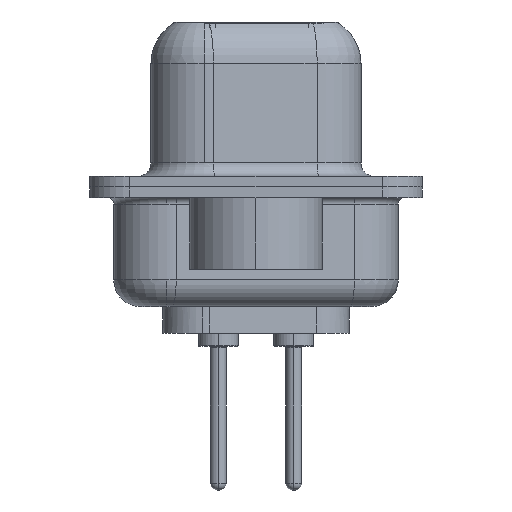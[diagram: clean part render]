
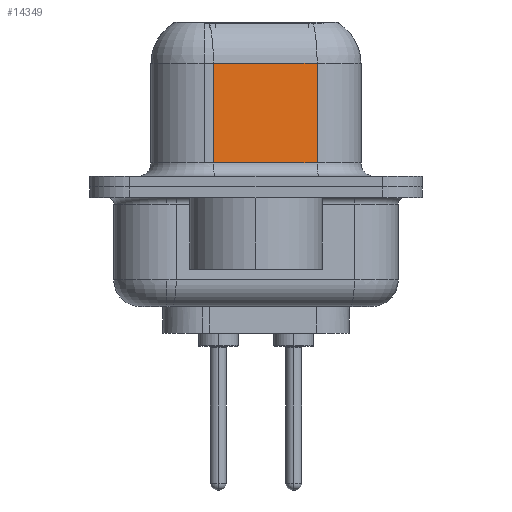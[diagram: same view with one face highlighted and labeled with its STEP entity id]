
A CAD part, left-side view. The second image highlights one B-rep face of the part: STEP entity #14349.
In plain terms, the highlighted planar face has unit normal (-0.985, -0.174, 0).
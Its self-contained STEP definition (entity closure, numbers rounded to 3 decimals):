
#186 = CARTESIAN_POINT ( 'NONE',  ( 4.355, 1.603, 4.65 ) ) ;
#962 = CARTESIAN_POINT ( 'NONE',  ( 4.355, 1.603, 6.4 ) ) ;
#1112 = VERTEX_POINT ( 'NONE', #186 ) ;
#1827 = EDGE_LOOP ( 'NONE', ( #10583, #21552, #18004, #3445 ) ) ;
#3055 = CARTESIAN_POINT ( 'NONE',  ( 5.043, -2.297, 0.9 ) ) ;
#3445 = ORIENTED_EDGE ( 'NONE', *, *, #12301, .T. ) ;
#4118 = FACE_OUTER_BOUND ( 'NONE', #1827, .T. ) ;
#4533 = VERTEX_POINT ( 'NONE', #3055 ) ;
#4885 = VERTEX_POINT ( 'NONE', #18457 ) ;
#5683 = DIRECTION ( 'NONE',  ( -0.174, 0.985, 0. ) ) ;
#7573 = LINE ( 'NONE', #21363, #15563 ) ;
#9321 = DIRECTION ( 'NONE',  ( 0.985, 0.174, 0. ) ) ;
#10583 = ORIENTED_EDGE ( 'NONE', *, *, #20795, .F. ) ;
#10875 = CARTESIAN_POINT ( 'NONE',  ( 5.043, -2.297, 6.4 ) ) ;
#12301 = EDGE_CURVE ( 'NONE', #4885, #4533, #7573, .T. ) ;
#12419 = CARTESIAN_POINT ( 'NONE',  ( 5.043, -2.297, 4.65 ) ) ;
#12812 = VECTOR ( 'NONE', #5683, 1000. ) ;
#12827 = AXIS2_PLACEMENT_3D ( 'NONE', #10875, #9321, #16061 ) ;
#14120 = LINE ( 'NONE', #962, #17999 ) ;
#14142 = EDGE_CURVE ( 'NONE', #16254, #1112, #20801, .T. ) ;
#14349 = ADVANCED_FACE ( 'NONE', ( #4118 ), #17700, .F. ) ;
#14574 = CARTESIAN_POINT ( 'NONE',  ( 5.043, -2.297, 4.65 ) ) ;
#15563 = VECTOR ( 'NONE', #17720, 1000. ) ;
#16061 = DIRECTION ( 'NONE',  ( -0.174, 0.985, 0. ) ) ;
#16108 = CARTESIAN_POINT ( 'NONE',  ( 5.043, -2.297, 6.4 ) ) ;
#16135 = EDGE_CURVE ( 'NONE', #1112, #4885, #14120, .T. ) ;
#16254 = VERTEX_POINT ( 'NONE', #14574 ) ;
#17700 = PLANE ( 'NONE',  #12827 ) ;
#17720 = DIRECTION ( 'NONE',  ( 0.174, -0.985, 0. ) ) ;
#17999 = VECTOR ( 'NONE', #20861, 1000. ) ;
#18004 = ORIENTED_EDGE ( 'NONE', *, *, #16135, .T. ) ;
#18457 = CARTESIAN_POINT ( 'NONE',  ( 4.355, 1.603, 0.9 ) ) ;
#18812 = VECTOR ( 'NONE', #19292, 1000. ) ;
#19292 = DIRECTION ( 'NONE',  ( 0., 0., -1. ) ) ;
#20795 = EDGE_CURVE ( 'NONE', #16254, #4533, #21164, .T. ) ;
#20801 = LINE ( 'NONE', #12419, #12812 ) ;
#20861 = DIRECTION ( 'NONE',  ( 0., 0., -1. ) ) ;
#21164 = LINE ( 'NONE', #16108, #18812 ) ;
#21363 = CARTESIAN_POINT ( 'NONE',  ( 5.043, -2.297, 0.9 ) ) ;
#21552 = ORIENTED_EDGE ( 'NONE', *, *, #14142, .T. ) ;
